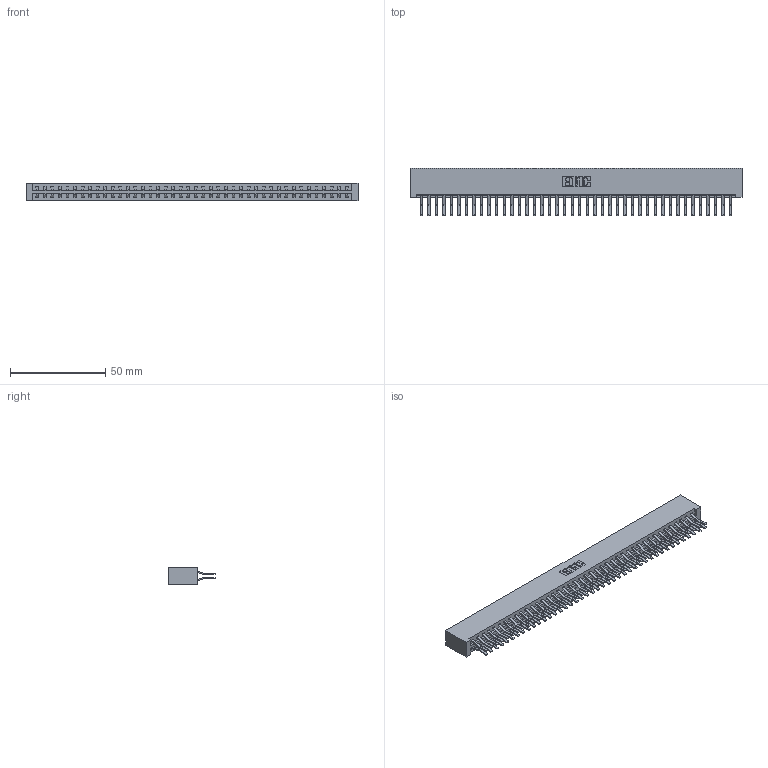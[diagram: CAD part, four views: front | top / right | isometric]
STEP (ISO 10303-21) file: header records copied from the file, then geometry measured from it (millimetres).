
FILE_DESCRIPTION (( 'STEP AP203' ), '1' );
FILE_NAME ('337-084-560-201.STEP', '2019-10-10T14:29:49', ( '' ), ( '' ), 'SwSTEP 2.0', 'SolidWorks 2016', '' );
FILE_SCHEMA (( 'CONFIG_CONTROL_DESIGN' ));
Length unit declared in the file: inch
Products named in the file (3): 337-084-560-201; 337 Part_No Mounting Lugs; 345-292-001_560 Tail
Assembly tree (85 placements, depth 2):
  337-084-560-201
    337 Part_No Mounting Lugs
    345-292-001_560 Tail  x84
Bounding box: 174.29 x 24.78 x 9.4 mm (x, y, z)
Volume: 19679.9 mm3; surface area: 23897.8 mm2
Topology: 85 solids, 85 shells, 4810 faces, 14315 edges, 9430 vertices
Faces by surface type: plane 3258, cylinder 1552
Entity records: 32375 total; most frequent: CARTESIAN_POINT 5454, ORIENTED_EDGE 5390, DIRECTION 4635, EDGE_CURVE 2695, VECTOR 2571, LINE 2571, VERTEX_POINT 1794, AXIS2_PLACEMENT_3D 1032
